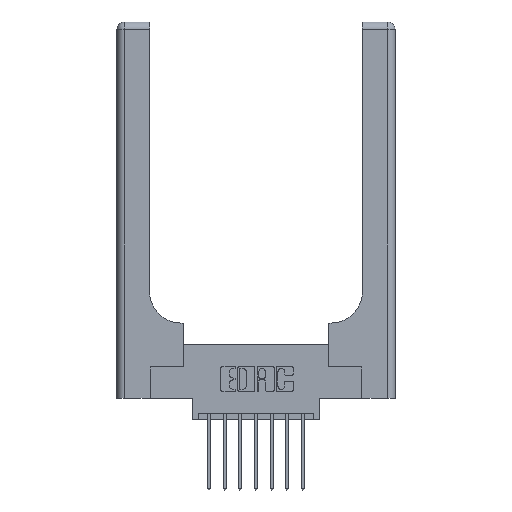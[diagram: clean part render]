
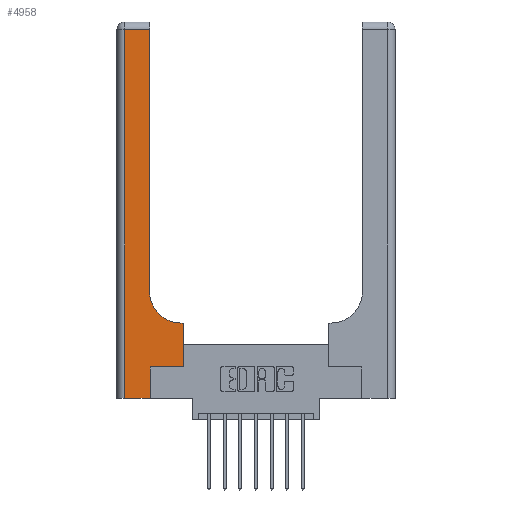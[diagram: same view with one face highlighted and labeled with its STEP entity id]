
A CAD part, top view. The second image highlights one B-rep face of the part: STEP entity #4958.
In plain terms, the highlighted planar face has unit normal (0, 0, 1).
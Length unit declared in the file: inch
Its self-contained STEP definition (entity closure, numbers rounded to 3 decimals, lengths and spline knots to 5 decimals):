
#345 = VERTEX_POINT ( 'NONE', #13216 ) ;
#437 = CARTESIAN_POINT ( 'NONE',  ( 0.26, 3., 0.37 ) ) ;
#509 = ORIENTED_EDGE ( 'NONE', *, *, #887, .T. ) ;
#589 = EDGE_CURVE ( 'NONE', #345, #9746, #10679, .T. ) ;
#653 = VERTEX_POINT ( 'NONE', #1296 ) ;
#674 = ORIENTED_EDGE ( 'NONE', *, *, #589, .T. ) ;
#767 = DIRECTION ( 'NONE',  ( 1., 0., 0. ) ) ;
#887 = EDGE_CURVE ( 'NONE', #9746, #4065, #12878, .T. ) ;
#1019 = LINE ( 'NONE', #9181, #6790 ) ;
#1044 = CARTESIAN_POINT ( 'NONE',  ( 0.06, 3., 0.37 ) ) ;
#1296 = CARTESIAN_POINT ( 'NONE',  ( 0.265, 0., 0.37 ) ) ;
#1827 = CARTESIAN_POINT ( 'NONE',  ( 0.51, 0.85, 0.37 ) ) ;
#1835 = VECTOR ( 'NONE', #14235, 39.37008 ) ;
#2435 = DIRECTION ( 'NONE',  ( -1., 0., 0. ) ) ;
#2516 = CARTESIAN_POINT ( 'NONE',  ( 0., 3., 0.37 ) ) ;
#2537 = ORIENTED_EDGE ( 'NONE', *, *, #5168, .T. ) ;
#2572 = LINE ( 'NONE', #10729, #1835 ) ;
#2689 = VECTOR ( 'NONE', #3945, 39.37008 ) ;
#2796 = CARTESIAN_POINT ( 'NONE',  ( 0.265, 0.25, 0.37 ) ) ;
#2868 = LINE ( 'NONE', #437, #7344 ) ;
#3219 = ORIENTED_EDGE ( 'NONE', *, *, #6803, .T. ) ;
#3302 = DIRECTION ( 'NONE',  ( 0., 1., 0. ) ) ;
#3360 = EDGE_CURVE ( 'NONE', #12281, #345, #1019, .T. ) ;
#3373 = CARTESIAN_POINT ( 'NONE',  ( 0.265, 0.25, 0.37 ) ) ;
#3605 = LINE ( 'NONE', #3373, #12773 ) ;
#3945 = DIRECTION ( 'NONE',  ( -1., 0., 0. ) ) ;
#4065 = VERTEX_POINT ( 'NONE', #13643 ) ;
#4468 = DIRECTION ( 'NONE',  ( 0., 1., 0. ) ) ;
#4958 = ADVANCED_FACE ( 'NONE', ( #7961 ), #10599, .F. ) ;
#5094 = LINE ( 'NONE', #10974, #2689 ) ;
#5168 = EDGE_CURVE ( 'NONE', #5659, #10799, #5094, .T. ) ;
#5659 = VERTEX_POINT ( 'NONE', #9039 ) ;
#5734 = VECTOR ( 'NONE', #4468, 39.37008 ) ;
#5781 = CARTESIAN_POINT ( 'NONE',  ( 0.06, 0., 0.37 ) ) ;
#5868 = CARTESIAN_POINT ( 'NONE',  ( 0.26, 0.6, 0.37 ) ) ;
#5872 = DIRECTION ( 'NONE',  ( -1., 0., 0. ) ) ;
#6458 = ORIENTED_EDGE ( 'NONE', *, *, #12973, .T. ) ;
#6478 = EDGE_CURVE ( 'NONE', #10799, #9450, #12209, .T. ) ;
#6790 = VECTOR ( 'NONE', #3302, 39.37008 ) ;
#6803 = EDGE_CURVE ( 'NONE', #4065, #5659, #2868, .T. ) ;
#7082 = AXIS2_PLACEMENT_3D ( 'NONE', #2516, #7182, #5872 ) ;
#7182 = DIRECTION ( 'NONE',  ( 0., 0., -1. ) ) ;
#7344 = VECTOR ( 'NONE', #11030, 39.37008 ) ;
#7744 = ORIENTED_EDGE ( 'NONE', *, *, #14167, .T. ) ;
#7961 = FACE_OUTER_BOUND ( 'NONE', #12687, .T. ) ;
#8713 = DIRECTION ( 'NONE',  ( 0., -1., 0. ) ) ;
#8998 = AXIS2_PLACEMENT_3D ( 'NONE', #1827, #13716, #767 ) ;
#9039 = CARTESIAN_POINT ( 'NONE',  ( 0.26, 2.94, 0.37 ) ) ;
#9064 = LINE ( 'NONE', #11352, #5734 ) ;
#9181 = CARTESIAN_POINT ( 'NONE',  ( 0.528, 0.25, 0.37 ) ) ;
#9450 = VERTEX_POINT ( 'NONE', #5781 ) ;
#9548 = VECTOR ( 'NONE', #8713, 39.37008 ) ;
#9746 = VERTEX_POINT ( 'NONE', #9886 ) ;
#9886 = CARTESIAN_POINT ( 'NONE',  ( 0.51, 0.6, 0.37 ) ) ;
#10599 = PLANE ( 'NONE',  #7082 ) ;
#10679 = LINE ( 'NONE', #5868, #11890 ) ;
#10729 = CARTESIAN_POINT ( 'NONE',  ( 0., 0., 0.37 ) ) ;
#10799 = VERTEX_POINT ( 'NONE', #10893 ) ;
#10893 = CARTESIAN_POINT ( 'NONE',  ( 0.06, 2.94, 0.37 ) ) ;
#10974 = CARTESIAN_POINT ( 'NONE',  ( 0., 2.94, 0.37 ) ) ;
#11030 = DIRECTION ( 'NONE',  ( 0., 1., 0. ) ) ;
#11352 = CARTESIAN_POINT ( 'NONE',  ( 0.265, 0., 0.37 ) ) ;
#11522 = EDGE_CURVE ( 'NONE', #13212, #12281, #3605, .T. ) ;
#11890 = VECTOR ( 'NONE', #2435, 39.37008 ) ;
#12209 = LINE ( 'NONE', #1044, #9548 ) ;
#12281 = VERTEX_POINT ( 'NONE', #14599 ) ;
#12687 = EDGE_LOOP ( 'NONE', ( #3219, #2537, #14175, #7744, #6458, #14302, #14243, #674, #509 ) ) ;
#12773 = VECTOR ( 'NONE', #12909, 39.37008 ) ;
#12878 = CIRCLE ( 'NONE', #8998, 0.25 ) ;
#12909 = DIRECTION ( 'NONE',  ( 1., 0., 0. ) ) ;
#12973 = EDGE_CURVE ( 'NONE', #653, #13212, #9064, .T. ) ;
#13212 = VERTEX_POINT ( 'NONE', #2796 ) ;
#13216 = CARTESIAN_POINT ( 'NONE',  ( 0.528, 0.6, 0.37 ) ) ;
#13643 = CARTESIAN_POINT ( 'NONE',  ( 0.26, 0.85, 0.37 ) ) ;
#13716 = DIRECTION ( 'NONE',  ( 0., 0., -1. ) ) ;
#14167 = EDGE_CURVE ( 'NONE', #9450, #653, #2572, .T. ) ;
#14175 = ORIENTED_EDGE ( 'NONE', *, *, #6478, .T. ) ;
#14235 = DIRECTION ( 'NONE',  ( 1., 0., 0. ) ) ;
#14243 = ORIENTED_EDGE ( 'NONE', *, *, #3360, .T. ) ;
#14302 = ORIENTED_EDGE ( 'NONE', *, *, #11522, .T. ) ;
#14599 = CARTESIAN_POINT ( 'NONE',  ( 0.528, 0.25, 0.37 ) ) ;
